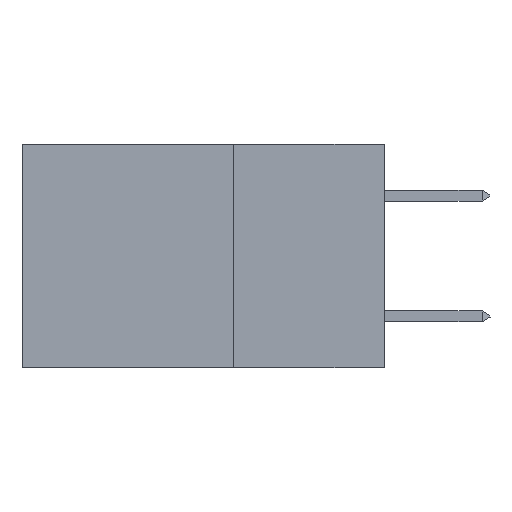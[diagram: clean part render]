
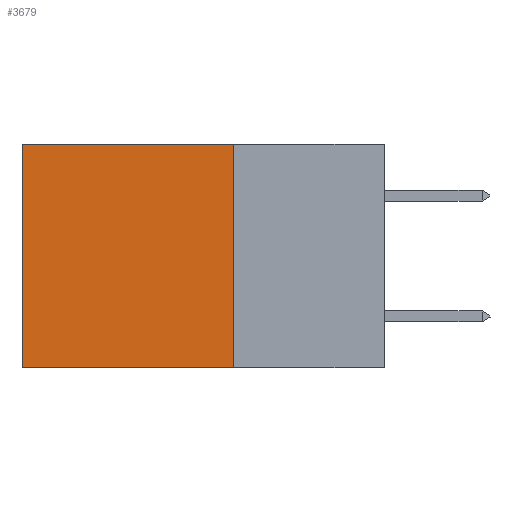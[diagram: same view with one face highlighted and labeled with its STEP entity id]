
A CAD part, left-side view. The second image highlights one B-rep face of the part: STEP entity #3679.
In plain terms, the highlighted planar face has unit normal (-1, 0, 0).
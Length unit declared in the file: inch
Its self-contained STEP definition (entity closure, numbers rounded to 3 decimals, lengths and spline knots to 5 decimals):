
#961 = DIRECTION ( 'NONE',  ( 1., 0., 0. ) ) ;
#1080 = ORIENTED_EDGE ( 'NONE', *, *, #13565, .F. ) ;
#1747 = CARTESIAN_POINT ( 'NONE',  ( 0.2875, 0.6, -0.37 ) ) ;
#1961 = ORIENTED_EDGE ( 'NONE', *, *, #15373, .T. ) ;
#2379 = CARTESIAN_POINT ( 'NONE',  ( 0.2875, 0.25, 0. ) ) ;
#2432 = VECTOR ( 'NONE', #5617, 39.37008 ) ;
#2455 = FACE_OUTER_BOUND ( 'NONE', #6601, .T. ) ;
#2816 = CARTESIAN_POINT ( 'NONE',  ( 0.2875, 0.25, 0. ) ) ;
#3140 = VECTOR ( 'NONE', #15614, 39.37008 ) ;
#3679 = ADVANCED_FACE ( 'NONE', ( #2455 ), #11421, .F. ) ;
#4386 = ORIENTED_EDGE ( 'NONE', *, *, #13468, .T. ) ;
#5177 = CARTESIAN_POINT ( 'NONE',  ( 0.2875, 0.25, 0. ) ) ;
#5277 = VERTEX_POINT ( 'NONE', #1747 ) ;
#5617 = DIRECTION ( 'NONE',  ( 0., 0., -1. ) ) ;
#5834 = LINE ( 'NONE', #13427, #2432 ) ;
#6435 = CARTESIAN_POINT ( 'NONE',  ( 0.2875, 0.25, -0.37 ) ) ;
#6601 = EDGE_LOOP ( 'NONE', ( #4386, #1080, #14509, #1961 ) ) ;
#7301 = VECTOR ( 'NONE', #10505, 39.37008 ) ;
#8626 = CARTESIAN_POINT ( 'NONE',  ( 0.2875, 0.25, 0. ) ) ;
#8915 = LINE ( 'NONE', #2816, #7301 ) ;
#9048 = VERTEX_POINT ( 'NONE', #2379 ) ;
#9108 = EDGE_CURVE ( 'NONE', #9048, #10070, #8915, .T. ) ;
#9215 = VECTOR ( 'NONE', #10896, 39.37008 ) ;
#9665 = CARTESIAN_POINT ( 'NONE',  ( 0.2875, 0.25, -0.37 ) ) ;
#9746 = VERTEX_POINT ( 'NONE', #12373 ) ;
#9917 = DIRECTION ( 'NONE',  ( 0., 0., -1. ) ) ;
#10070 = VERTEX_POINT ( 'NONE', #6435 ) ;
#10505 = DIRECTION ( 'NONE',  ( 0., 0., -1. ) ) ;
#10839 = LINE ( 'NONE', #9665, #9215 ) ;
#10896 = DIRECTION ( 'NONE',  ( 0., 1., 0. ) ) ;
#11421 = PLANE ( 'NONE',  #14439 ) ;
#12373 = CARTESIAN_POINT ( 'NONE',  ( 0.2875, 0.6, 0. ) ) ;
#12469 = LINE ( 'NONE', #5177, #3140 ) ;
#13427 = CARTESIAN_POINT ( 'NONE',  ( 0.2875, 0.6, 0. ) ) ;
#13468 = EDGE_CURVE ( 'NONE', #9746, #5277, #5834, .T. ) ;
#13565 = EDGE_CURVE ( 'NONE', #10070, #5277, #10839, .T. ) ;
#14439 = AXIS2_PLACEMENT_3D ( 'NONE', #8626, #961, #9917 ) ;
#14509 = ORIENTED_EDGE ( 'NONE', *, *, #9108, .F. ) ;
#15373 = EDGE_CURVE ( 'NONE', #9048, #9746, #12469, .T. ) ;
#15614 = DIRECTION ( 'NONE',  ( 0., 1., 0. ) ) ;
